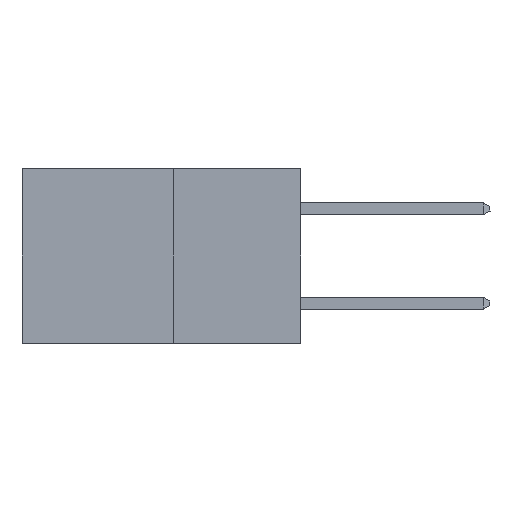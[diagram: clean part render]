
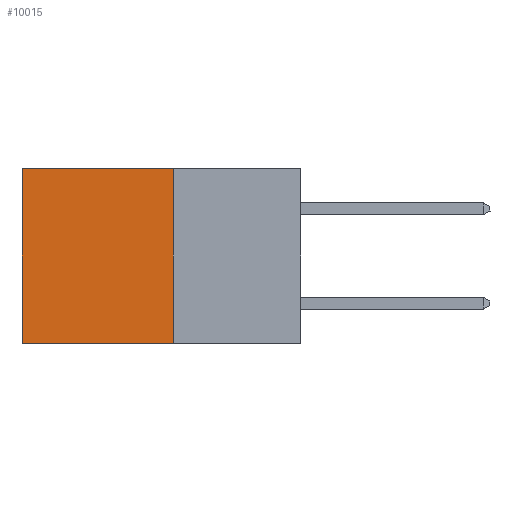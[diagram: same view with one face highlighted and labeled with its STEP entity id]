
A CAD part, left-side view. The second image highlights one B-rep face of the part: STEP entity #10015.
In plain terms, the highlighted planar face has unit normal (-1, 0, 0).
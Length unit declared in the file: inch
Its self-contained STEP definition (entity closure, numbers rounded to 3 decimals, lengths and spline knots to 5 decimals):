
#140 = VECTOR ( 'NONE', #15642, 39.37008 ) ;
#1367 = EDGE_CURVE ( 'NONE', #15230, #2553, #4243, .T. ) ;
#2000 = EDGE_LOOP ( 'NONE', ( #6115, #11026, #3165, #15959 ) ) ;
#2553 = VERTEX_POINT ( 'NONE', #16538 ) ;
#3165 = ORIENTED_EDGE ( 'NONE', *, *, #17815, .F. ) ;
#3174 = LINE ( 'NONE', #10587, #13734 ) ;
#3463 = EDGE_CURVE ( 'NONE', #14661, #2553, #14309, .T. ) ;
#4243 = LINE ( 'NONE', #9147, #15225 ) ;
#6115 = ORIENTED_EDGE ( 'NONE', *, *, #1367, .T. ) ;
#6832 = AXIS2_PLACEMENT_3D ( 'NONE', #8220, #13070, #11895 ) ;
#7925 = LINE ( 'NONE', #15723, #140 ) ;
#8220 = CARTESIAN_POINT ( 'NONE',  ( 0.277, 0.27, -0.37 ) ) ;
#8421 = VERTEX_POINT ( 'NONE', #11879 ) ;
#9147 = CARTESIAN_POINT ( 'NONE',  ( 0.277, 0.59, -0.37 ) ) ;
#10015 = ADVANCED_FACE ( 'NONE', ( #17316 ), #12890, .F. ) ;
#10176 = EDGE_CURVE ( 'NONE', #8421, #15230, #3174, .T. ) ;
#10587 = CARTESIAN_POINT ( 'NONE',  ( 0.277, 0.27, 0. ) ) ;
#10608 = DIRECTION ( 'NONE',  ( 0., 0., -1. ) ) ;
#11026 = ORIENTED_EDGE ( 'NONE', *, *, #3463, .F. ) ;
#11567 = CARTESIAN_POINT ( 'NONE',  ( 0.277, 0.59, 0. ) ) ;
#11879 = CARTESIAN_POINT ( 'NONE',  ( 0.277, 0.27, 0. ) ) ;
#11895 = DIRECTION ( 'NONE',  ( 0., 0., -1. ) ) ;
#12890 = PLANE ( 'NONE',  #6832 ) ;
#13070 = DIRECTION ( 'NONE',  ( 1., 0., 0. ) ) ;
#13734 = VECTOR ( 'NONE', #13895, 39.37008 ) ;
#13895 = DIRECTION ( 'NONE',  ( 0., 1., 0. ) ) ;
#14178 = CARTESIAN_POINT ( 'NONE',  ( 0.277, 0.27, -0.37 ) ) ;
#14195 = DIRECTION ( 'NONE',  ( 0., 1., 0. ) ) ;
#14309 = LINE ( 'NONE', #14178, #18126 ) ;
#14661 = VERTEX_POINT ( 'NONE', #16752 ) ;
#15225 = VECTOR ( 'NONE', #10608, 39.37008 ) ;
#15230 = VERTEX_POINT ( 'NONE', #11567 ) ;
#15642 = DIRECTION ( 'NONE',  ( 0., 0., -1. ) ) ;
#15723 = CARTESIAN_POINT ( 'NONE',  ( 0.277, 0.27, -0.37 ) ) ;
#15959 = ORIENTED_EDGE ( 'NONE', *, *, #10176, .T. ) ;
#16538 = CARTESIAN_POINT ( 'NONE',  ( 0.277, 0.59, -0.37 ) ) ;
#16752 = CARTESIAN_POINT ( 'NONE',  ( 0.277, 0.27, -0.37 ) ) ;
#17316 = FACE_OUTER_BOUND ( 'NONE', #2000, .T. ) ;
#17815 = EDGE_CURVE ( 'NONE', #8421, #14661, #7925, .T. ) ;
#18126 = VECTOR ( 'NONE', #14195, 39.37008 ) ;
